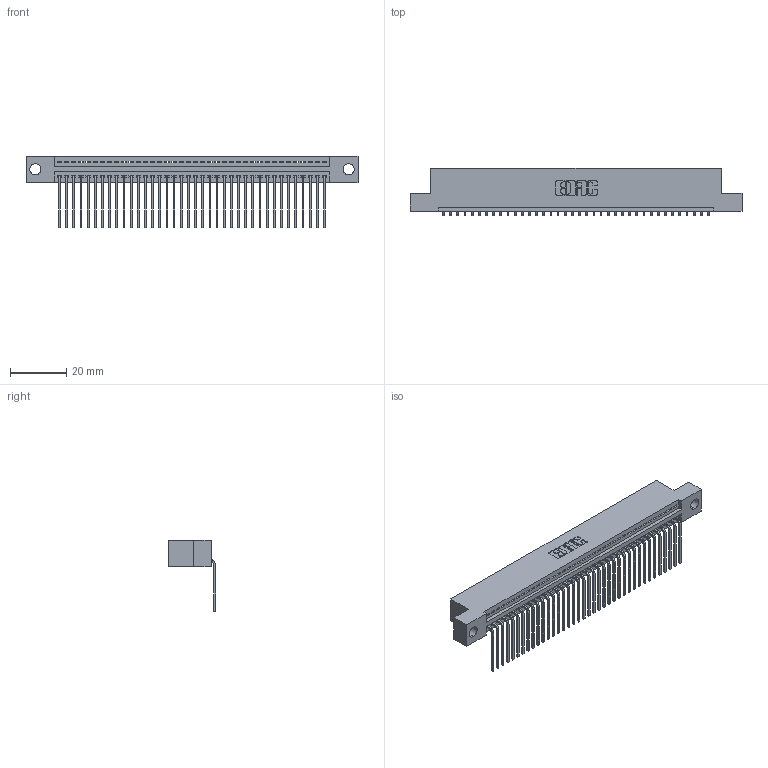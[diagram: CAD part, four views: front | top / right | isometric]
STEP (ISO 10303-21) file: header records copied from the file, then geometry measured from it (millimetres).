
FILE_DESCRIPTION (( 'STEP AP203' ), '1' );
FILE_NAME ('345-038-559-104.STEP', '2018-08-30T10:17:57', ( '' ), ( '' ), 'SwSTEP 2.0', 'SolidWorks 2016', '' );
FILE_SCHEMA (( 'CONFIG_CONTROL_DESIGN' ));
Length unit declared in the file: inch
Products named in the file (3): 345-292-001_558 559 Tail - 1; 345-038-559-104; 345 Part_Flush Mounting Lugs - 0.156 Dia-TH
Assembly tree (39 placements, depth 2):
  345-038-559-104
    345 Part_Flush Mounting Lugs - 0.156 Dia-TH
    345-292-001_558 559 Tail - 1  x38
Bounding box: 117.73 x 16.75 x 25.53 mm (x, y, z)
Volume: 11188 mm3; surface area: 15366.2 mm2
Topology: 39 solids, 39 shells, 2406 faces, 7257 edges, 4786 vertices
Faces by surface type: plane 1676, cylinder 730
Entity records: 29225 total; most frequent: CARTESIAN_POINT 5070, ORIENTED_EDGE 5042, DIRECTION 4433, EDGE_CURVE 2521, VECTOR 2237, LINE 2237, VERTEX_POINT 1678, AXIS2_PLACEMENT_3D 1098
